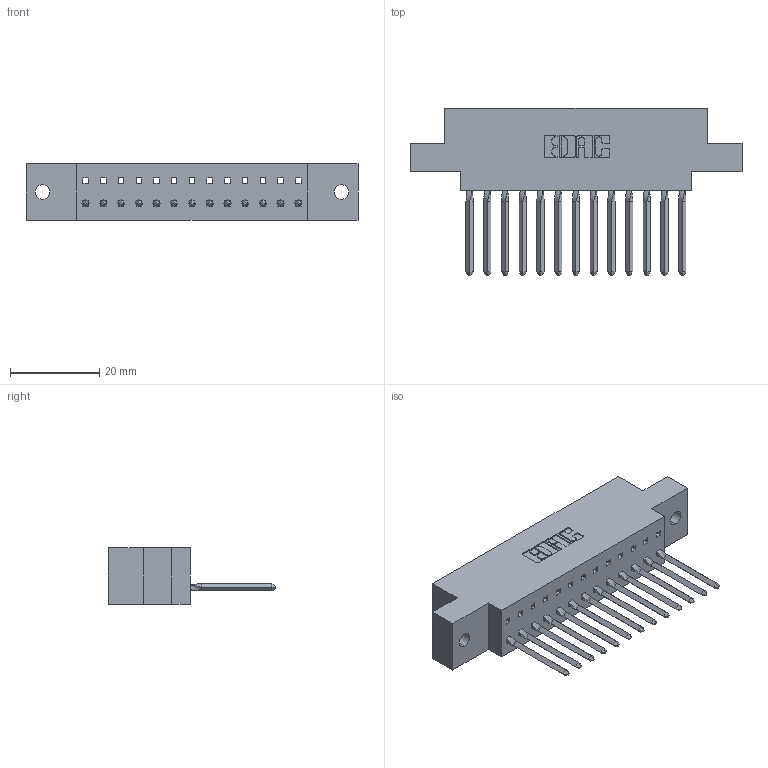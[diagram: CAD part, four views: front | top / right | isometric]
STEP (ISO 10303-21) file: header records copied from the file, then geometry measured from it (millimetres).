
FILE_DESCRIPTION (( 'STEP AP203' ), '1' );
FILE_NAME ('317-013-542-602.STEP', '2020-02-27T14:19:31', ( '' ), ( '' ), 'SwSTEP 2.0', 'SolidWorks 2016', '' );
FILE_SCHEMA (( 'CONFIG_CONTROL_DESIGN' ));
Length unit declared in the file: inch
Products named in the file (3): 317-013-542-602; 317 Part_.144 Dia; 317-290-003_542
Assembly tree (14 placements, depth 2):
  317-013-542-602
    317 Part_.144 Dia
    317-290-003_542  x13
Bounding box: 74.22 x 37.34 x 12.7 mm (x, y, z)
Volume: 10657 mm3; surface area: 12079.7 mm2
Topology: 14 solids, 14 shells, 1077 faces, 3096 edges, 2002 vertices
Faces by surface type: plane 890, cylinder 135, bspline 52
Entity records: 21441 total; most frequent: CARTESIAN_POINT 4044, ORIENTED_EDGE 3720, DIRECTION 3154, EDGE_CURVE 1860, LINE 1690, VECTOR 1690, VERTEX_POINT 1234, AXIS2_PLACEMENT_3D 732
